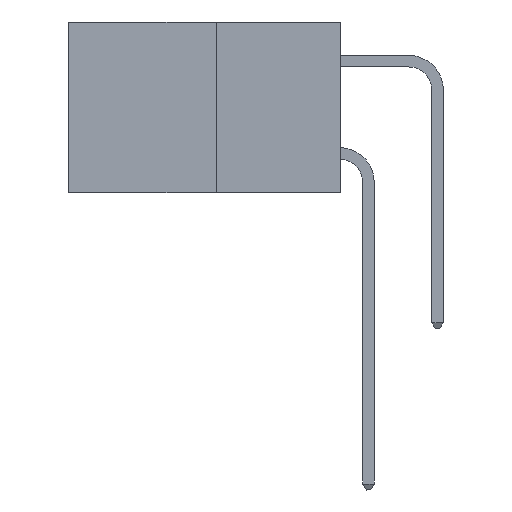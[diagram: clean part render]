
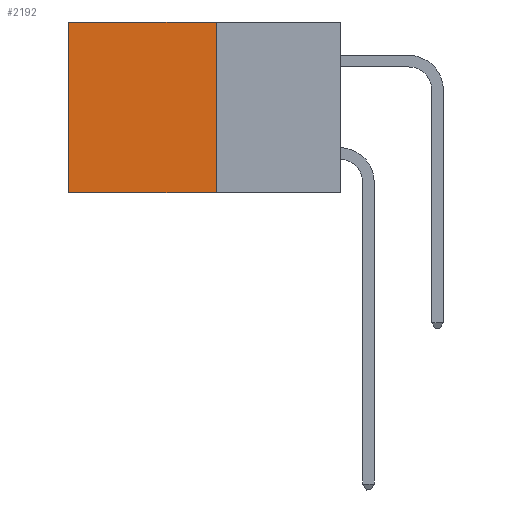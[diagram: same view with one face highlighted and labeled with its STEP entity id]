
A CAD part, left-side view. The second image highlights one B-rep face of the part: STEP entity #2192.
In plain terms, the highlighted planar face has unit normal (-1, 0, 0).
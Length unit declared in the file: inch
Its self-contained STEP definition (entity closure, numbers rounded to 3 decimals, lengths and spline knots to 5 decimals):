
#1687 = VERTEX_POINT ( 'NONE', #20804 ) ;
#2110 = ORIENTED_EDGE ( 'NONE', *, *, #7919, .F. ) ;
#2192 = ADVANCED_FACE ( 'NONE', ( #10755 ), #6989, .F. ) ;
#2522 = VERTEX_POINT ( 'NONE', #4351 ) ;
#3650 = VERTEX_POINT ( 'NONE', #3972 ) ;
#3972 = CARTESIAN_POINT ( 'NONE',  ( 0.277, 0.27, -0.37 ) ) ;
#4351 = CARTESIAN_POINT ( 'NONE',  ( 0.277, 0.59, -0.37 ) ) ;
#4475 = DIRECTION ( 'NONE',  ( 0., 0., -1. ) ) ;
#5141 = LINE ( 'NONE', #8734, #13623 ) ;
#5691 = VECTOR ( 'NONE', #12997, 39.37008 ) ;
#6209 = ORIENTED_EDGE ( 'NONE', *, *, #16985, .T. ) ;
#6966 = DIRECTION ( 'NONE',  ( 0., 0., -1. ) ) ;
#6971 = DIRECTION ( 'NONE',  ( 1., 0., 0. ) ) ;
#6989 = PLANE ( 'NONE',  #19079 ) ;
#7036 = EDGE_CURVE ( 'NONE', #12070, #2522, #9088, .T. ) ;
#7060 = DIRECTION ( 'NONE',  ( 0., 1., 0. ) ) ;
#7919 = EDGE_CURVE ( 'NONE', #3650, #2522, #5141, .T. ) ;
#8734 = CARTESIAN_POINT ( 'NONE',  ( 0.277, 0.27, -0.37 ) ) ;
#9005 = CARTESIAN_POINT ( 'NONE',  ( 0.277, 0.27, -0.37 ) ) ;
#9088 = LINE ( 'NONE', #19974, #17630 ) ;
#10369 = VECTOR ( 'NONE', #19136, 39.37008 ) ;
#10695 = CARTESIAN_POINT ( 'NONE',  ( 0.277, 0.27, 0. ) ) ;
#10755 = FACE_OUTER_BOUND ( 'NONE', #17748, .T. ) ;
#12070 = VERTEX_POINT ( 'NONE', #12510 ) ;
#12510 = CARTESIAN_POINT ( 'NONE',  ( 0.277, 0.59, 0. ) ) ;
#12965 = EDGE_CURVE ( 'NONE', #1687, #3650, #19166, .T. ) ;
#12997 = DIRECTION ( 'NONE',  ( 0., 0., -1. ) ) ;
#13623 = VECTOR ( 'NONE', #7060, 39.37008 ) ;
#16985 = EDGE_CURVE ( 'NONE', #1687, #12070, #19351, .T. ) ;
#17630 = VECTOR ( 'NONE', #4475, 39.37008 ) ;
#17748 = EDGE_LOOP ( 'NONE', ( #18079, #2110, #19724, #6209 ) ) ;
#18079 = ORIENTED_EDGE ( 'NONE', *, *, #7036, .T. ) ;
#19079 = AXIS2_PLACEMENT_3D ( 'NONE', #9005, #6971, #6966 ) ;
#19136 = DIRECTION ( 'NONE',  ( 0., 1., 0. ) ) ;
#19166 = LINE ( 'NONE', #19649, #5691 ) ;
#19351 = LINE ( 'NONE', #10695, #10369 ) ;
#19649 = CARTESIAN_POINT ( 'NONE',  ( 0.277, 0.27, -0.37 ) ) ;
#19724 = ORIENTED_EDGE ( 'NONE', *, *, #12965, .F. ) ;
#19974 = CARTESIAN_POINT ( 'NONE',  ( 0.277, 0.59, -0.37 ) ) ;
#20804 = CARTESIAN_POINT ( 'NONE',  ( 0.277, 0.27, 0. ) ) ;
